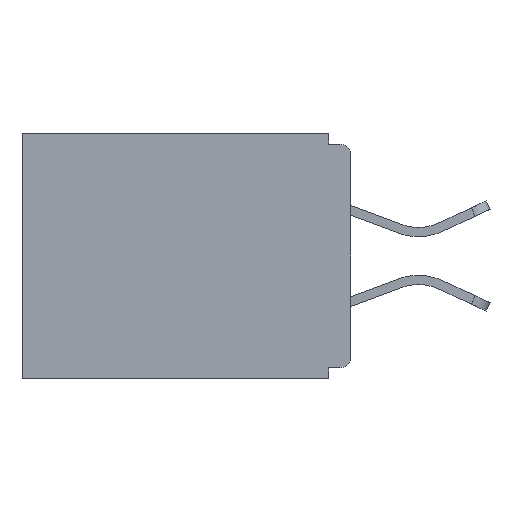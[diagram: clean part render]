
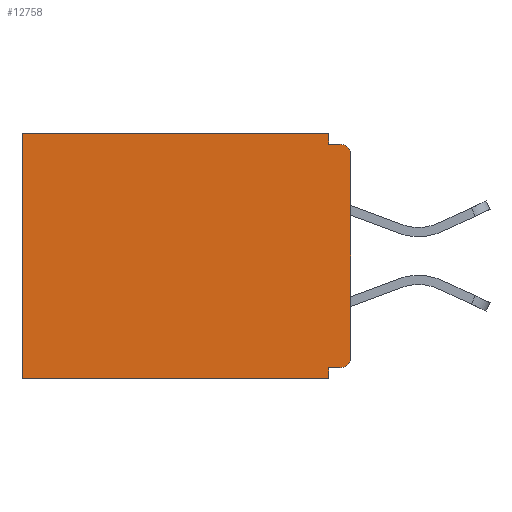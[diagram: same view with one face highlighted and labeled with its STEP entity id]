
A CAD part, left-side view. The second image highlights one B-rep face of the part: STEP entity #12758.
In plain terms, the highlighted planar face has unit normal (-1, 0, 0).
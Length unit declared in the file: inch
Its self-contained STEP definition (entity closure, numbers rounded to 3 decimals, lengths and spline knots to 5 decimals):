
#193 = DIRECTION ( 'NONE',  ( -1., 0., 0. ) ) ;
#207 = CARTESIAN_POINT ( 'NONE',  ( 0.298, 0., 0. ) ) ;
#635 = CARTESIAN_POINT ( 'NONE',  ( 0.298, 0.015, -0.328 ) ) ;
#746 = ORIENTED_EDGE ( 'NONE', *, *, #17263, .F. ) ;
#751 = VECTOR ( 'NONE', #9820, 39.37008 ) ;
#1067 = LINE ( 'NONE', #11627, #9388 ) ;
#1135 = VERTEX_POINT ( 'NONE', #13784 ) ;
#1144 = EDGE_CURVE ( 'NONE', #9028, #12393, #12610, .T. ) ;
#1159 = AXIS2_PLACEMENT_3D ( 'NONE', #11119, #193, #5835 ) ;
#1543 = ORIENTED_EDGE ( 'NONE', *, *, #9635, .F. ) ;
#1608 = PLANE ( 'NONE',  #12918 ) ;
#1879 = DIRECTION ( 'NONE',  ( 0., 0., -1. ) ) ;
#2133 = CARTESIAN_POINT ( 'NONE',  ( 0.298, 0.031, -0.015 ) ) ;
#2270 = AXIS2_PLACEMENT_3D ( 'NONE', #11513, #12764, #1879 ) ;
#3477 = VERTEX_POINT ( 'NONE', #15771 ) ;
#3765 = VECTOR ( 'NONE', #7596, 39.37008 ) ;
#4448 = VERTEX_POINT ( 'NONE', #7004 ) ;
#4546 = ORIENTED_EDGE ( 'NONE', *, *, #6927, .F. ) ;
#4663 = LINE ( 'NONE', #15502, #5710 ) ;
#4886 = DIRECTION ( 'NONE',  ( 0., 1., 0. ) ) ;
#5125 = CIRCLE ( 'NONE', #2270, 0.015 ) ;
#5179 = CARTESIAN_POINT ( 'NONE',  ( 0.298, 0., -0.015 ) ) ;
#5669 = CARTESIAN_POINT ( 'NONE',  ( 0.298, 0., -0.03 ) ) ;
#5710 = VECTOR ( 'NONE', #14072, 39.37008 ) ;
#5835 = DIRECTION ( 'NONE',  ( 0., 0., -1. ) ) ;
#6023 = CARTESIAN_POINT ( 'NONE',  ( 0.298, 0.46, 0. ) ) ;
#6326 = LINE ( 'NONE', #6023, #3765 ) ;
#6381 = VERTEX_POINT ( 'NONE', #11025 ) ;
#6927 = EDGE_CURVE ( 'NONE', #9028, #8781, #4663, .T. ) ;
#6980 = CARTESIAN_POINT ( 'NONE',  ( 0.298, 0., 0. ) ) ;
#7004 = CARTESIAN_POINT ( 'NONE',  ( 0.298, 0.46, -0.343 ) ) ;
#7121 = ORIENTED_EDGE ( 'NONE', *, *, #10263, .T. ) ;
#7192 = VECTOR ( 'NONE', #12417, 39.37008 ) ;
#7466 = VERTEX_POINT ( 'NONE', #10186 ) ;
#7571 = CARTESIAN_POINT ( 'NONE',  ( 0.298, 0.46, 0. ) ) ;
#7587 = ORIENTED_EDGE ( 'NONE', *, *, #11928, .T. ) ;
#7596 = DIRECTION ( 'NONE',  ( 0., 0., -1. ) ) ;
#7696 = LINE ( 'NONE', #6980, #14376 ) ;
#8781 = VERTEX_POINT ( 'NONE', #2133 ) ;
#8820 = EDGE_CURVE ( 'NONE', #12009, #6381, #1067, .T. ) ;
#8829 = CARTESIAN_POINT ( 'NONE',  ( 0.298, 0., 0. ) ) ;
#9028 = VERTEX_POINT ( 'NONE', #16317 ) ;
#9388 = VECTOR ( 'NONE', #4886, 39.37008 ) ;
#9470 = EDGE_CURVE ( 'NONE', #8781, #3477, #12073, .T. ) ;
#9490 = DIRECTION ( 'NONE',  ( 0., 0., -1. ) ) ;
#9505 = CIRCLE ( 'NONE', #1159, 0.015 ) ;
#9635 = EDGE_CURVE ( 'NONE', #16353, #7466, #7696, .T. ) ;
#9686 = ORIENTED_EDGE ( 'NONE', *, *, #9470, .F. ) ;
#9820 = DIRECTION ( 'NONE',  ( 0., 1., 0. ) ) ;
#9840 = ORIENTED_EDGE ( 'NONE', *, *, #15466, .T. ) ;
#10186 = CARTESIAN_POINT ( 'NONE',  ( 0.298, 0., -0.313 ) ) ;
#10263 = EDGE_CURVE ( 'NONE', #12009, #7466, #5125, .T. ) ;
#11025 = CARTESIAN_POINT ( 'NONE',  ( 0.298, 0.031, -0.328 ) ) ;
#11056 = CARTESIAN_POINT ( 'NONE',  ( 0.298, 0.031, -0.343 ) ) ;
#11119 = CARTESIAN_POINT ( 'NONE',  ( 0.298, 0.015, -0.03 ) ) ;
#11334 = VECTOR ( 'NONE', #11588, 39.37008 ) ;
#11359 = CARTESIAN_POINT ( 'NONE',  ( 0.298, 0., -0.343 ) ) ;
#11513 = CARTESIAN_POINT ( 'NONE',  ( 0.298, 0.015, -0.313 ) ) ;
#11588 = DIRECTION ( 'NONE',  ( 0., 1., 0. ) ) ;
#11627 = CARTESIAN_POINT ( 'NONE',  ( 0.298, 0., -0.328 ) ) ;
#11777 = ORIENTED_EDGE ( 'NONE', *, *, #8820, .F. ) ;
#11928 = EDGE_CURVE ( 'NONE', #12393, #4448, #6326, .T. ) ;
#12009 = VERTEX_POINT ( 'NONE', #635 ) ;
#12073 = LINE ( 'NONE', #5179, #15211 ) ;
#12274 = EDGE_LOOP ( 'NONE', ( #9840, #9686, #4546, #16210, #7587, #746, #14978, #11777, #7121, #1543 ) ) ;
#12393 = VERTEX_POINT ( 'NONE', #7571 ) ;
#12417 = DIRECTION ( 'NONE',  ( 0., 0., -1. ) ) ;
#12610 = LINE ( 'NONE', #207, #751 ) ;
#12758 = ADVANCED_FACE ( 'NONE', ( #14921 ), #1608, .F. ) ;
#12764 = DIRECTION ( 'NONE',  ( -1., 0., 0. ) ) ;
#12918 = AXIS2_PLACEMENT_3D ( 'NONE', #8829, #15454, #16746 ) ;
#13784 = CARTESIAN_POINT ( 'NONE',  ( 0.298, 0.031, -0.343 ) ) ;
#14072 = DIRECTION ( 'NONE',  ( 0., 0., -1. ) ) ;
#14376 = VECTOR ( 'NONE', #9490, 39.37008 ) ;
#14469 = LINE ( 'NONE', #11359, #11334 ) ;
#14921 = FACE_OUTER_BOUND ( 'NONE', #12274, .T. ) ;
#14978 = ORIENTED_EDGE ( 'NONE', *, *, #15497, .F. ) ;
#15211 = VECTOR ( 'NONE', #16308, 39.37008 ) ;
#15454 = DIRECTION ( 'NONE',  ( 1., 0., 0. ) ) ;
#15466 = EDGE_CURVE ( 'NONE', #16353, #3477, #9505, .T. ) ;
#15497 = EDGE_CURVE ( 'NONE', #6381, #1135, #16640, .T. ) ;
#15502 = CARTESIAN_POINT ( 'NONE',  ( 0.298, 0.031, -0.343 ) ) ;
#15771 = CARTESIAN_POINT ( 'NONE',  ( 0.298, 0.015, -0.015 ) ) ;
#16210 = ORIENTED_EDGE ( 'NONE', *, *, #1144, .T. ) ;
#16308 = DIRECTION ( 'NONE',  ( 0., -1., 0. ) ) ;
#16317 = CARTESIAN_POINT ( 'NONE',  ( 0.298, 0.031, 0. ) ) ;
#16353 = VERTEX_POINT ( 'NONE', #5669 ) ;
#16640 = LINE ( 'NONE', #11056, #7192 ) ;
#16746 = DIRECTION ( 'NONE',  ( 0., 0., -1. ) ) ;
#17263 = EDGE_CURVE ( 'NONE', #1135, #4448, #14469, .T. ) ;
